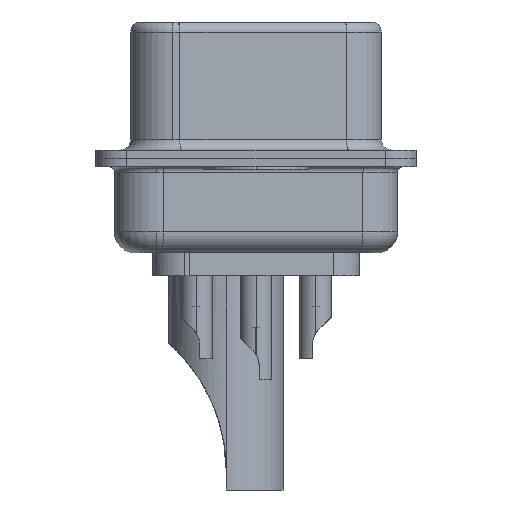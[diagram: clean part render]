
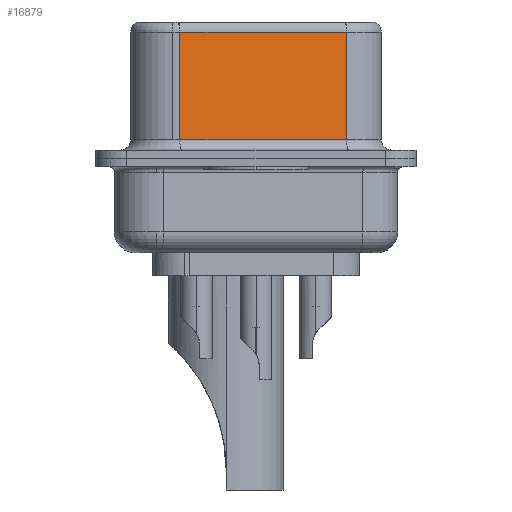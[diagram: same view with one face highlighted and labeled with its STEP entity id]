
A CAD part, left-side view. The second image highlights one B-rep face of the part: STEP entity #16879.
In plain terms, the highlighted planar face has unit normal (-0.985, -0.174, 0).
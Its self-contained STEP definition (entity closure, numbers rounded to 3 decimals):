
#332 = EDGE_CURVE ( 'NONE', #6110, #16865, #23199, .T. ) ;
#1167 = CARTESIAN_POINT ( 'NONE',  ( 5.132, -4.322, 6.52 ) ) ;
#1280 = ORIENTED_EDGE ( 'NONE', *, *, #9276, .F. ) ;
#3091 = EDGE_CURVE ( 'NONE', #12061, #6110, #20627, .T. ) ;
#3225 = CARTESIAN_POINT ( 'NONE',  ( 5.132, -4.322, 0.9 ) ) ;
#3278 = VECTOR ( 'NONE', #24163, 1000. ) ;
#3387 = ORIENTED_EDGE ( 'NONE', *, *, #15357, .T. ) ;
#3568 = CARTESIAN_POINT ( 'NONE',  ( 5.132, -4.322, 6.02 ) ) ;
#4108 = VECTOR ( 'NONE', #25801, 1000. ) ;
#4366 = CARTESIAN_POINT ( 'NONE',  ( 5.132, -4.322, 6.02 ) ) ;
#6110 = VERTEX_POINT ( 'NONE', #14938 ) ;
#7474 = VECTOR ( 'NONE', #10445, 1000. ) ;
#7511 = DIRECTION ( 'NONE',  ( 0.985, 0.174, 0. ) ) ;
#9276 = EDGE_CURVE ( 'NONE', #18641, #16865, #9423, .T. ) ;
#9423 = LINE ( 'NONE', #9746, #3278 ) ;
#9746 = CARTESIAN_POINT ( 'NONE',  ( 5.132, -4.322, 6.52 ) ) ;
#10306 = VECTOR ( 'NONE', #21447, 1000. ) ;
#10445 = DIRECTION ( 'NONE',  ( -0.174, 0.985, 0. ) ) ;
#10884 = FACE_OUTER_BOUND ( 'NONE', #11213, .T. ) ;
#11213 = EDGE_LOOP ( 'NONE', ( #1280, #3387, #20346, #16589 ) ) ;
#12061 = VERTEX_POINT ( 'NONE', #25986 ) ;
#12977 = LINE ( 'NONE', #4366, #7474 ) ;
#13089 = CARTESIAN_POINT ( 'NONE',  ( 3.73, 3.628, 6.52 ) ) ;
#14618 = CARTESIAN_POINT ( 'NONE',  ( 5.132, -4.322, 0.9 ) ) ;
#14938 = CARTESIAN_POINT ( 'NONE',  ( 3.73, 3.628, 0.9 ) ) ;
#15357 = EDGE_CURVE ( 'NONE', #18641, #12061, #12977, .T. ) ;
#16589 = ORIENTED_EDGE ( 'NONE', *, *, #332, .T. ) ;
#16865 = VERTEX_POINT ( 'NONE', #3225 ) ;
#16879 = ADVANCED_FACE ( 'NONE', ( #10884 ), #23859, .F. ) ;
#18641 = VERTEX_POINT ( 'NONE', #3568 ) ;
#20346 = ORIENTED_EDGE ( 'NONE', *, *, #3091, .T. ) ;
#20627 = LINE ( 'NONE', #13089, #4108 ) ;
#21447 = DIRECTION ( 'NONE',  ( 0.174, -0.985, 0. ) ) ;
#21913 = DIRECTION ( 'NONE',  ( -0.174, 0.985, 0. ) ) ;
#23199 = LINE ( 'NONE', #14618, #10306 ) ;
#23859 = PLANE ( 'NONE',  #25766 ) ;
#24163 = DIRECTION ( 'NONE',  ( 0., 0., -1. ) ) ;
#25766 = AXIS2_PLACEMENT_3D ( 'NONE', #1167, #7511, #21913 ) ;
#25801 = DIRECTION ( 'NONE',  ( 0., 0., -1. ) ) ;
#25986 = CARTESIAN_POINT ( 'NONE',  ( 3.73, 3.628, 6.02 ) ) ;
